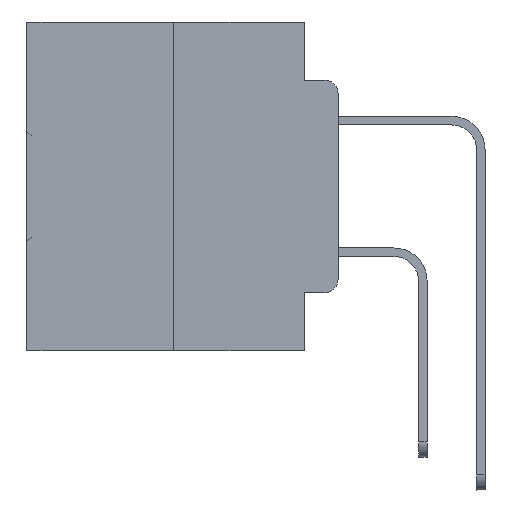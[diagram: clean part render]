
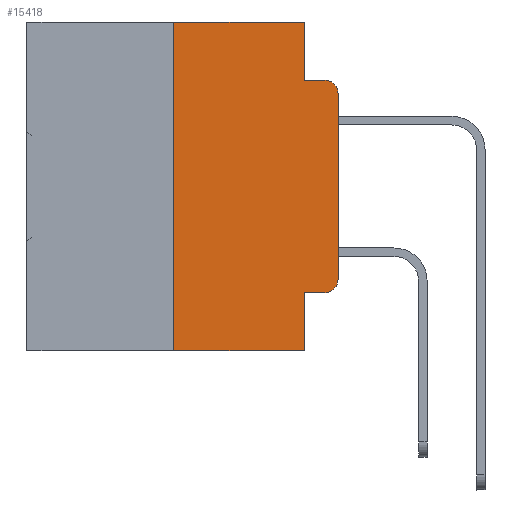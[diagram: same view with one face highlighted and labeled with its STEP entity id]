
A CAD part, left-side view. The second image highlights one B-rep face of the part: STEP entity #15418.
In plain terms, the highlighted planar face has unit normal (-1, 0, 0).
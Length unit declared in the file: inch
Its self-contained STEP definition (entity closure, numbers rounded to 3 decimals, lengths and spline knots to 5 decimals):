
#1428 = DIRECTION ( 'NONE',  ( -1., 0., 0. ) ) ;
#1450 = CARTESIAN_POINT ( 'NONE',  ( 0., 0.25, -0.5 ) ) ;
#2321 = ORIENTED_EDGE ( 'NONE', *, *, #7103, .F. ) ;
#2842 = CARTESIAN_POINT ( 'NONE',  ( 0., 0.051, -0.0885 ) ) ;
#4079 = ORIENTED_EDGE ( 'NONE', *, *, #23797, .T. ) ;
#4149 = DIRECTION ( 'NONE',  ( -1., 0., 0. ) ) ;
#4718 = CARTESIAN_POINT ( 'NONE',  ( 0., 0.051, -0.0885 ) ) ;
#5296 = CARTESIAN_POINT ( 'NONE',  ( 0., 0.25, 0. ) ) ;
#6505 = VERTEX_POINT ( 'NONE', #11514 ) ;
#6810 = LINE ( 'NONE', #33273, #27848 ) ;
#7103 = EDGE_CURVE ( 'NONE', #27430, #8083, #33524, .T. ) ;
#7493 = VECTOR ( 'NONE', #9145, 39.37008 ) ;
#8083 = VERTEX_POINT ( 'NONE', #4718 ) ;
#8988 = CARTESIAN_POINT ( 'NONE',  ( 0., 0.02, -0.0885 ) ) ;
#9145 = DIRECTION ( 'NONE',  ( 0., -1., 0. ) ) ;
#10565 = CARTESIAN_POINT ( 'NONE',  ( 0., 0.02, -0.4115 ) ) ;
#11514 = CARTESIAN_POINT ( 'NONE',  ( 0., 0.051, -0.5 ) ) ;
#12331 = LINE ( 'NONE', #2842, #33903 ) ;
#12508 = LINE ( 'NONE', #5296, #33238 ) ;
#12529 = CARTESIAN_POINT ( 'NONE',  ( 0., 0.473, 0. ) ) ;
#12654 = DIRECTION ( 'NONE',  ( 0., 0., -1. ) ) ;
#12902 = EDGE_LOOP ( 'NONE', ( #30257, #4079, #26485, #2321, #25604, #33228, #30987, #13441, #14235, #21209 ) ) ;
#13441 = ORIENTED_EDGE ( 'NONE', *, *, #33311, .F. ) ;
#13914 = DIRECTION ( 'NONE',  ( 0., 0., -1. ) ) ;
#14235 = ORIENTED_EDGE ( 'NONE', *, *, #26239, .T. ) ;
#14480 = VECTOR ( 'NONE', #17471, 39.37008 ) ;
#14558 = EDGE_CURVE ( 'NONE', #8083, #28842, #12331, .T. ) ;
#15241 = CARTESIAN_POINT ( 'NONE',  ( 0., 0.25, 0. ) ) ;
#15376 = FACE_OUTER_BOUND ( 'NONE', #12902, .T. ) ;
#15418 = ADVANCED_FACE ( 'NONE', ( #15376 ), #23627, .F. ) ;
#15987 = VERTEX_POINT ( 'NONE', #34218 ) ;
#16759 = CIRCLE ( 'NONE', #25766, 0.02 ) ;
#17204 = DIRECTION ( 'NONE',  ( 0., -1., 0. ) ) ;
#17394 = EDGE_CURVE ( 'NONE', #29008, #6505, #24276, .T. ) ;
#17471 = DIRECTION ( 'NONE',  ( 0., 0., 1. ) ) ;
#18077 = CARTESIAN_POINT ( 'NONE',  ( 0., 0.02, -0.3915 ) ) ;
#19291 = VECTOR ( 'NONE', #28069, 39.37008 ) ;
#19470 = DIRECTION ( 'NONE',  ( 0., -1., 0. ) ) ;
#20757 = CARTESIAN_POINT ( 'NONE',  ( 0., 0.02, -0.1085 ) ) ;
#20837 = DIRECTION ( 'NONE',  ( 0., 0., -1. ) ) ;
#21209 = ORIENTED_EDGE ( 'NONE', *, *, #24459, .T. ) ;
#21352 = LINE ( 'NONE', #33592, #7493 ) ;
#21687 = DIRECTION ( 'NONE',  ( 0., -1., 0. ) ) ;
#21822 = LINE ( 'NONE', #28233, #14480 ) ;
#22955 = EDGE_CURVE ( 'NONE', #31463, #27430, #6810, .T. ) ;
#23507 = DIRECTION ( 'NONE',  ( 0., 0., -1. ) ) ;
#23627 = PLANE ( 'NONE',  #27607 ) ;
#23797 = EDGE_CURVE ( 'NONE', #30510, #28842, #16759, .T. ) ;
#23819 = AXIS2_PLACEMENT_3D ( 'NONE', #18077, #1428, #20837 ) ;
#24276 = LINE ( 'NONE', #29768, #28846 ) ;
#24459 = EDGE_CURVE ( 'NONE', #32304, #15987, #29814, .T. ) ;
#24832 = CARTESIAN_POINT ( 'NONE',  ( 0., 0.051, 0. ) ) ;
#25282 = CARTESIAN_POINT ( 'NONE',  ( 0., 0.051, 0. ) ) ;
#25420 = VECTOR ( 'NONE', #13914, 39.37008 ) ;
#25572 = EDGE_CURVE ( 'NONE', #15987, #30510, #21822, .T. ) ;
#25604 = ORIENTED_EDGE ( 'NONE', *, *, #22955, .F. ) ;
#25766 = AXIS2_PLACEMENT_3D ( 'NONE', #20757, #4149, #23507 ) ;
#26239 = EDGE_CURVE ( 'NONE', #29316, #32304, #21352, .T. ) ;
#26485 = ORIENTED_EDGE ( 'NONE', *, *, #14558, .F. ) ;
#27295 = DIRECTION ( 'NONE',  ( 0., 0., 1. ) ) ;
#27430 = VERTEX_POINT ( 'NONE', #31128 ) ;
#27432 = CARTESIAN_POINT ( 'NONE',  ( 0., 0.051, -0.4115 ) ) ;
#27607 = AXIS2_PLACEMENT_3D ( 'NONE', #12529, #28977, #12654 ) ;
#27848 = VECTOR ( 'NONE', #17204, 39.37008 ) ;
#28069 = DIRECTION ( 'NONE',  ( 0., 0., -1. ) ) ;
#28233 = CARTESIAN_POINT ( 'NONE',  ( 0., 0., 0. ) ) ;
#28842 = VERTEX_POINT ( 'NONE', #8988 ) ;
#28846 = VECTOR ( 'NONE', #21687, 39.37008 ) ;
#28977 = DIRECTION ( 'NONE',  ( 1., 0., 0. ) ) ;
#29008 = VERTEX_POINT ( 'NONE', #1450 ) ;
#29316 = VERTEX_POINT ( 'NONE', #27432 ) ;
#29768 = CARTESIAN_POINT ( 'NONE',  ( 0., 0.473, -0.5 ) ) ;
#29814 = CIRCLE ( 'NONE', #23819, 0.02 ) ;
#30257 = ORIENTED_EDGE ( 'NONE', *, *, #25572, .T. ) ;
#30510 = VERTEX_POINT ( 'NONE', #35266 ) ;
#30987 = ORIENTED_EDGE ( 'NONE', *, *, #17394, .T. ) ;
#31128 = CARTESIAN_POINT ( 'NONE',  ( 0., 0.051, 0. ) ) ;
#31463 = VERTEX_POINT ( 'NONE', #15241 ) ;
#32304 = VERTEX_POINT ( 'NONE', #10565 ) ;
#32444 = LINE ( 'NONE', #24832, #25420 ) ;
#33228 = ORIENTED_EDGE ( 'NONE', *, *, #35070, .F. ) ;
#33238 = VECTOR ( 'NONE', #27295, 39.37008 ) ;
#33273 = CARTESIAN_POINT ( 'NONE',  ( 0., 0.473, 0. ) ) ;
#33311 = EDGE_CURVE ( 'NONE', #29316, #6505, #32444, .T. ) ;
#33524 = LINE ( 'NONE', #25282, #19291 ) ;
#33592 = CARTESIAN_POINT ( 'NONE',  ( 0., 0.051, -0.4115 ) ) ;
#33903 = VECTOR ( 'NONE', #19470, 39.37008 ) ;
#34218 = CARTESIAN_POINT ( 'NONE',  ( 0., 0., -0.3915 ) ) ;
#35070 = EDGE_CURVE ( 'NONE', #29008, #31463, #12508, .T. ) ;
#35266 = CARTESIAN_POINT ( 'NONE',  ( 0., 0., -0.1085 ) ) ;
